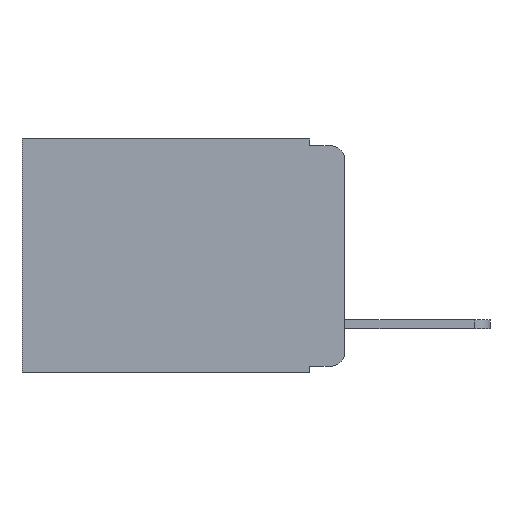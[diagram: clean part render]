
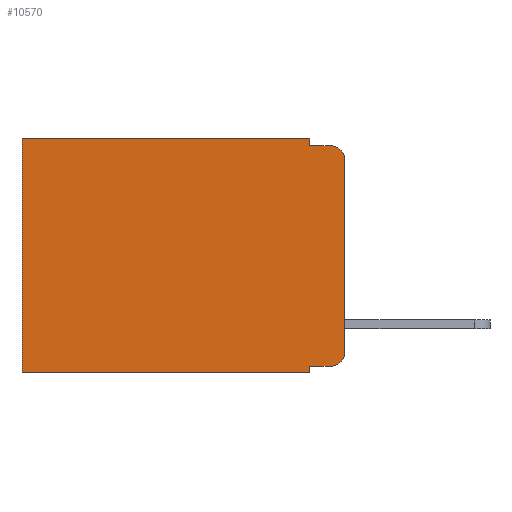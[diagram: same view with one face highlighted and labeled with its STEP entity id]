
A CAD part, left-side view. The second image highlights one B-rep face of the part: STEP entity #10570.
In plain terms, the highlighted planar face has unit normal (-1, 0, 0).
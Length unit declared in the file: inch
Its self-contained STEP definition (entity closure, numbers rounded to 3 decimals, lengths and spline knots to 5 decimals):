
#14 = CARTESIAN_POINT ( 'NONE',  ( 0.298, 0., 0. ) ) ;
#72 = LINE ( 'NONE', #3368, #6369 ) ;
#168 = EDGE_CURVE ( 'NONE', #14282, #5421, #12071, .T. ) ;
#482 = VERTEX_POINT ( 'NONE', #5625 ) ;
#489 = AXIS2_PLACEMENT_3D ( 'NONE', #11778, #15658, #7871 ) ;
#524 = ORIENTED_EDGE ( 'NONE', *, *, #12857, .F. ) ;
#743 = ORIENTED_EDGE ( 'NONE', *, *, #4999, .T. ) ;
#923 = ORIENTED_EDGE ( 'NONE', *, *, #5500, .T. ) ;
#940 = ORIENTED_EDGE ( 'NONE', *, *, #15330, .F. ) ;
#1165 = VECTOR ( 'NONE', #11521, 39.37008 ) ;
#1388 = DIRECTION ( 'NONE',  ( 0., 0., -1. ) ) ;
#1689 = CARTESIAN_POINT ( 'NONE',  ( 0.298, 0.051, -0.01 ) ) ;
#2052 = LINE ( 'NONE', #10026, #14560 ) ;
#2174 = EDGE_CURVE ( 'NONE', #8682, #4478, #4697, .T. ) ;
#2253 = ORIENTED_EDGE ( 'NONE', *, *, #2174, .T. ) ;
#2406 = CARTESIAN_POINT ( 'NONE',  ( 0.298, 0.02, -0.01 ) ) ;
#2432 = EDGE_CURVE ( 'NONE', #6390, #482, #4493, .T. ) ;
#2435 = VECTOR ( 'NONE', #6575, 39.37008 ) ;
#2949 = CARTESIAN_POINT ( 'NONE',  ( 0.298, 0.02, -0.03 ) ) ;
#2955 = FACE_OUTER_BOUND ( 'NONE', #10231, .T. ) ;
#3154 = EDGE_CURVE ( 'NONE', #4478, #3247, #7184, .T. ) ;
#3247 = VERTEX_POINT ( 'NONE', #15048 ) ;
#3368 = CARTESIAN_POINT ( 'NONE',  ( 0.298, 0., 0. ) ) ;
#3854 = DIRECTION ( 'NONE',  ( 1., 0., 0. ) ) ;
#3923 = DIRECTION ( 'NONE',  ( 0., 1., 0. ) ) ;
#4131 = CARTESIAN_POINT ( 'NONE',  ( 0.298, 0.02, -0.333 ) ) ;
#4478 = VERTEX_POINT ( 'NONE', #4131 ) ;
#4493 = LINE ( 'NONE', #11334, #1165 ) ;
#4697 = LINE ( 'NONE', #9302, #13934 ) ;
#4956 = ORIENTED_EDGE ( 'NONE', *, *, #168, .T. ) ;
#4999 = EDGE_CURVE ( 'NONE', #13507, #482, #6564, .T. ) ;
#5079 = VERTEX_POINT ( 'NONE', #11360 ) ;
#5351 = LINE ( 'NONE', #1689, #8625 ) ;
#5421 = VERTEX_POINT ( 'NONE', #2406 ) ;
#5446 = DIRECTION ( 'NONE',  ( 0., 0., -1. ) ) ;
#5500 = EDGE_CURVE ( 'NONE', #5079, #13507, #2052, .T. ) ;
#5625 = CARTESIAN_POINT ( 'NONE',  ( 0.298, 0.473, -0.343 ) ) ;
#5643 = VECTOR ( 'NONE', #5446, 39.37008 ) ;
#5763 = LINE ( 'NONE', #13747, #2435 ) ;
#6175 = VECTOR ( 'NONE', #1388, 39.37008 ) ;
#6369 = VECTOR ( 'NONE', #7043, 39.37008 ) ;
#6390 = VERTEX_POINT ( 'NONE', #9265 ) ;
#6564 = LINE ( 'NONE', #8632, #6175 ) ;
#6575 = DIRECTION ( 'NONE',  ( 0., 0., -1. ) ) ;
#6610 = CARTESIAN_POINT ( 'NONE',  ( 0.298, 0., -0.03 ) ) ;
#7043 = DIRECTION ( 'NONE',  ( 0., 0., -1. ) ) ;
#7184 = CIRCLE ( 'NONE', #489, 0.02 ) ;
#7411 = CARTESIAN_POINT ( 'NONE',  ( 0.298, 0.051, -0.333 ) ) ;
#7711 = EDGE_CURVE ( 'NONE', #14282, #3247, #72, .T. ) ;
#7747 = AXIS2_PLACEMENT_3D ( 'NONE', #14, #3854, #12368 ) ;
#7871 = DIRECTION ( 'NONE',  ( 0., 0., -1. ) ) ;
#8040 = ORIENTED_EDGE ( 'NONE', *, *, #8921, .F. ) ;
#8447 = DIRECTION ( 'NONE',  ( 0., -1., 0. ) ) ;
#8625 = VECTOR ( 'NONE', #9112, 39.37008 ) ;
#8632 = CARTESIAN_POINT ( 'NONE',  ( 0.298, 0.473, 0. ) ) ;
#8682 = VERTEX_POINT ( 'NONE', #7411 ) ;
#8689 = PLANE ( 'NONE',  #7747 ) ;
#8921 = EDGE_CURVE ( 'NONE', #14415, #5421, #5351, .T. ) ;
#9112 = DIRECTION ( 'NONE',  ( 0., -1., 0. ) ) ;
#9265 = CARTESIAN_POINT ( 'NONE',  ( 0.298, 0.051, -0.343 ) ) ;
#9302 = CARTESIAN_POINT ( 'NONE',  ( 0.298, 0.051, -0.333 ) ) ;
#9503 = AXIS2_PLACEMENT_3D ( 'NONE', #2949, #13973, #14033 ) ;
#10026 = CARTESIAN_POINT ( 'NONE',  ( 0.298, 0., 0. ) ) ;
#10231 = EDGE_LOOP ( 'NONE', ( #13291, #4956, #8040, #940, #923, #743, #11720, #524, #2253, #15012 ) ) ;
#10339 = CARTESIAN_POINT ( 'NONE',  ( 0.298, 0.051, 0. ) ) ;
#10570 = ADVANCED_FACE ( 'NONE', ( #2955 ), #8689, .F. ) ;
#10621 = CARTESIAN_POINT ( 'NONE',  ( 0.298, 0.051, -0.01 ) ) ;
#11334 = CARTESIAN_POINT ( 'NONE',  ( 0.298, 0., -0.343 ) ) ;
#11360 = CARTESIAN_POINT ( 'NONE',  ( 0.298, 0.051, 0. ) ) ;
#11521 = DIRECTION ( 'NONE',  ( 0., 1., 0. ) ) ;
#11720 = ORIENTED_EDGE ( 'NONE', *, *, #2432, .F. ) ;
#11778 = CARTESIAN_POINT ( 'NONE',  ( 0.298, 0.02, -0.313 ) ) ;
#12071 = CIRCLE ( 'NONE', #9503, 0.02 ) ;
#12368 = DIRECTION ( 'NONE',  ( 0., 0., -1. ) ) ;
#12857 = EDGE_CURVE ( 'NONE', #8682, #6390, #15165, .T. ) ;
#13291 = ORIENTED_EDGE ( 'NONE', *, *, #7711, .F. ) ;
#13507 = VERTEX_POINT ( 'NONE', #15731 ) ;
#13747 = CARTESIAN_POINT ( 'NONE',  ( 0.298, 0.051, 0. ) ) ;
#13934 = VECTOR ( 'NONE', #8447, 39.37008 ) ;
#13973 = DIRECTION ( 'NONE',  ( -1., 0., 0. ) ) ;
#14033 = DIRECTION ( 'NONE',  ( 0., 0., -1. ) ) ;
#14282 = VERTEX_POINT ( 'NONE', #6610 ) ;
#14415 = VERTEX_POINT ( 'NONE', #10621 ) ;
#14560 = VECTOR ( 'NONE', #3923, 39.37008 ) ;
#15012 = ORIENTED_EDGE ( 'NONE', *, *, #3154, .T. ) ;
#15048 = CARTESIAN_POINT ( 'NONE',  ( 0.298, 0., -0.313 ) ) ;
#15165 = LINE ( 'NONE', #10339, #5643 ) ;
#15330 = EDGE_CURVE ( 'NONE', #5079, #14415, #5763, .T. ) ;
#15658 = DIRECTION ( 'NONE',  ( -1., 0., 0. ) ) ;
#15731 = CARTESIAN_POINT ( 'NONE',  ( 0.298, 0.473, 0. ) ) ;
